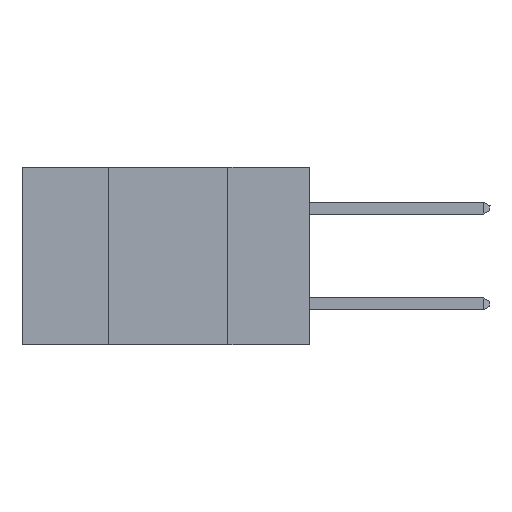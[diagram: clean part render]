
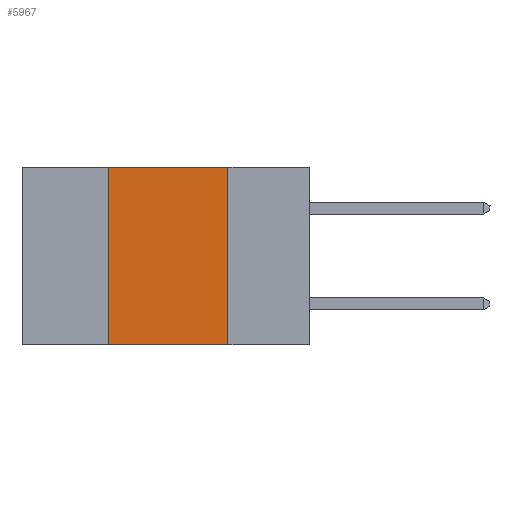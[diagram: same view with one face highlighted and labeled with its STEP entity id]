
A CAD part, left-side view. The second image highlights one B-rep face of the part: STEP entity #5967.
In plain terms, the highlighted planar face has unit normal (-1, 0, 0).
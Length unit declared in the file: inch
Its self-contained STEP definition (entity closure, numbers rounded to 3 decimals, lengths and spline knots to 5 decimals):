
#159 = DIRECTION ( 'NONE',  ( 1., 0., 0. ) ) ;
#474 = CARTESIAN_POINT ( 'NONE',  ( 0., 0.17, 0. ) ) ;
#734 = VERTEX_POINT ( 'NONE', #9293 ) ;
#892 = DIRECTION ( 'NONE',  ( 0., -1., 0. ) ) ;
#1017 = ORIENTED_EDGE ( 'NONE', *, *, #12738, .T. ) ;
#1603 = FACE_OUTER_BOUND ( 'NONE', #7314, .T. ) ;
#1691 = EDGE_CURVE ( 'NONE', #3686, #12455, #9378, .T. ) ;
#2360 = LINE ( 'NONE', #9612, #7293 ) ;
#3108 = CARTESIAN_POINT ( 'NONE',  ( 0., 0.6, 0. ) ) ;
#3686 = VERTEX_POINT ( 'NONE', #6226 ) ;
#3909 = VECTOR ( 'NONE', #10191, 39.37008 ) ;
#3954 = VECTOR ( 'NONE', #892, 39.37008 ) ;
#4204 = EDGE_CURVE ( 'NONE', #734, #3686, #9328, .T. ) ;
#4345 = AXIS2_PLACEMENT_3D ( 'NONE', #7098, #159, #9352 ) ;
#4829 = DIRECTION ( 'NONE',  ( 0., 0., -1. ) ) ;
#5047 = EDGE_CURVE ( 'NONE', #12455, #9175, #2360, .T. ) ;
#5967 = ADVANCED_FACE ( 'NONE', ( #1603 ), #11778, .F. ) ;
#6226 = CARTESIAN_POINT ( 'NONE',  ( 0., 0.42, 0. ) ) ;
#6600 = VECTOR ( 'NONE', #8458, 39.37008 ) ;
#6920 = LINE ( 'NONE', #7451, #6600 ) ;
#6939 = ORIENTED_EDGE ( 'NONE', *, *, #5047, .F. ) ;
#7098 = CARTESIAN_POINT ( 'NONE',  ( 0., 0.6, 0. ) ) ;
#7293 = VECTOR ( 'NONE', #4829, 39.37008 ) ;
#7314 = EDGE_LOOP ( 'NONE', ( #6939, #10831, #13255, #1017 ) ) ;
#7451 = CARTESIAN_POINT ( 'NONE',  ( 0., 0.6, -0.37 ) ) ;
#8458 = DIRECTION ( 'NONE',  ( 0., -1., 0. ) ) ;
#9175 = VERTEX_POINT ( 'NONE', #13531 ) ;
#9293 = CARTESIAN_POINT ( 'NONE',  ( 0., 0.42, -0.37 ) ) ;
#9328 = LINE ( 'NONE', #13259, #3909 ) ;
#9352 = DIRECTION ( 'NONE',  ( 0., 0., -1. ) ) ;
#9378 = LINE ( 'NONE', #3108, #3954 ) ;
#9612 = CARTESIAN_POINT ( 'NONE',  ( 0., 0.17, 0. ) ) ;
#10191 = DIRECTION ( 'NONE',  ( 0., 0., 1. ) ) ;
#10831 = ORIENTED_EDGE ( 'NONE', *, *, #1691, .F. ) ;
#11778 = PLANE ( 'NONE',  #4345 ) ;
#12455 = VERTEX_POINT ( 'NONE', #474 ) ;
#12738 = EDGE_CURVE ( 'NONE', #734, #9175, #6920, .T. ) ;
#13255 = ORIENTED_EDGE ( 'NONE', *, *, #4204, .F. ) ;
#13259 = CARTESIAN_POINT ( 'NONE',  ( 0., 0.42, 0. ) ) ;
#13531 = CARTESIAN_POINT ( 'NONE',  ( 0., 0.17, -0.37 ) ) ;
